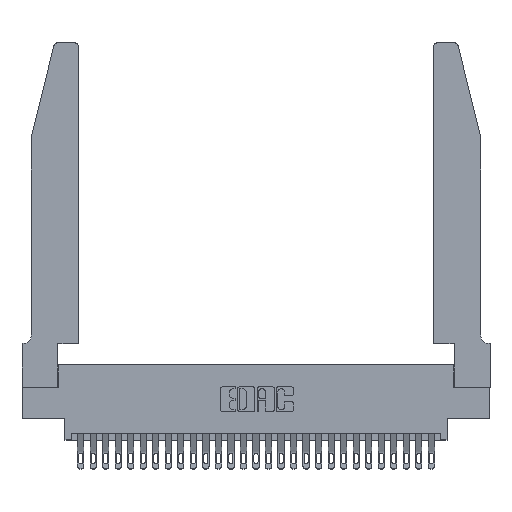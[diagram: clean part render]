
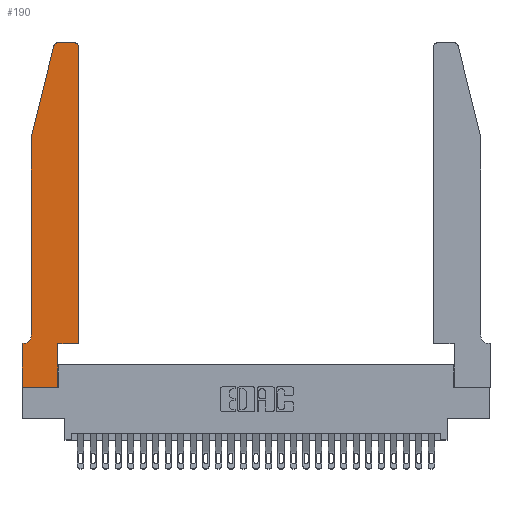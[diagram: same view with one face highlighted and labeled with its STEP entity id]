
A CAD part, top view. The second image highlights one B-rep face of the part: STEP entity #190.
In plain terms, the highlighted planar face has unit normal (0, 0, 1).
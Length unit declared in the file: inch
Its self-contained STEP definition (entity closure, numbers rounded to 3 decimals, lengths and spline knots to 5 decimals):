
#25 = ORIENTED_EDGE ( 'NONE', *, *, #14336, .T. ) ;
#148 = ORIENTED_EDGE ( 'NONE', *, *, #8840, .T. ) ;
#163 = EDGE_CURVE ( 'NONE', #23841, #16520, #17546, .T. ) ;
#190 = ADVANCED_FACE ( 'NONE', ( #3991 ), #472, .T. ) ;
#430 = VECTOR ( 'NONE', #6743, 39.37008 ) ;
#472 = PLANE ( 'NONE',  #8886 ) ;
#648 = CARTESIAN_POINT ( 'NONE',  ( 0.4505, 0.35, 0.37 ) ) ;
#1099 = EDGE_CURVE ( 'NONE', #1543, #5972, #5007, .T. ) ;
#1498 = LINE ( 'NONE', #7025, #430 ) ;
#1543 = VERTEX_POINT ( 'NONE', #26610 ) ;
#1707 = CARTESIAN_POINT ( 'NONE',  ( 0.2605, 2.75, 0.37 ) ) ;
#2311 = DIRECTION ( 'NONE',  ( 1., 0., 0. ) ) ;
#2401 = ORIENTED_EDGE ( 'NONE', *, *, #26664, .T. ) ;
#3390 = VECTOR ( 'NONE', #27976, 39.37008 ) ;
#3510 = DIRECTION ( 'NONE',  ( 0., 0., 1. ) ) ;
#3991 = FACE_OUTER_BOUND ( 'NONE', #22065, .T. ) ;
#4996 = EDGE_CURVE ( 'NONE', #13910, #7833, #11927, .T. ) ;
#5005 = CARTESIAN_POINT ( 'NONE',  ( 0.0755, 0.35, 0.37 ) ) ;
#5007 = CIRCLE ( 'NONE', #23324, 0.07 ) ;
#5354 = CIRCLE ( 'NONE', #14340, 0.03 ) ;
#5479 = VERTEX_POINT ( 'NONE', #13765 ) ;
#5972 = VERTEX_POINT ( 'NONE', #24914 ) ;
#6438 = DIRECTION ( 'NONE',  ( 0., -1., 0. ) ) ;
#6489 = VERTEX_POINT ( 'NONE', #14662 ) ;
#6595 = CARTESIAN_POINT ( 'NONE',  ( 0., 0.35, 0.37 ) ) ;
#6743 = DIRECTION ( 'NONE',  ( 0., -1., 0. ) ) ;
#6972 = EDGE_CURVE ( 'NONE', #5479, #14205, #20443, .T. ) ;
#7025 = CARTESIAN_POINT ( 'NONE',  ( 0., 0., 0.37 ) ) ;
#7113 = LINE ( 'NONE', #24559, #20734 ) ;
#7833 = VERTEX_POINT ( 'NONE', #26004 ) ;
#8429 = VECTOR ( 'NONE', #21575, 39.37008 ) ;
#8840 = EDGE_CURVE ( 'NONE', #16288, #6489, #14554, .T. ) ;
#8886 = AXIS2_PLACEMENT_3D ( 'NONE', #12289, #14259, #19126 ) ;
#8894 = EDGE_CURVE ( 'NONE', #14205, #1543, #14892, .T. ) ;
#8908 = CARTESIAN_POINT ( 'NONE',  ( 0.0055, 0.42, 0.37 ) ) ;
#9817 = EDGE_CURVE ( 'NONE', #5972, #24705, #28520, .T. ) ;
#9888 = CARTESIAN_POINT ( 'NONE',  ( 0., 0., 0.37 ) ) ;
#11049 = CARTESIAN_POINT ( 'NONE',  ( 0.0755, 2., 0.37 ) ) ;
#11228 = DIRECTION ( 'NONE',  ( 0., 0., -1. ) ) ;
#11453 = ORIENTED_EDGE ( 'NONE', *, *, #4996, .T. ) ;
#11559 = VECTOR ( 'NONE', #13982, 39.37008 ) ;
#11583 = DIRECTION ( 'NONE',  ( 0., 1., 0. ) ) ;
#11827 = DIRECTION ( 'NONE',  ( 1., 0., 0. ) ) ;
#11927 = LINE ( 'NONE', #13743, #27342 ) ;
#11958 = CARTESIAN_POINT ( 'NONE',  ( 0.2865, 0.35, 0.37 ) ) ;
#12289 = CARTESIAN_POINT ( 'NONE',  ( 0., 0.35, 0.37 ) ) ;
#12913 = CARTESIAN_POINT ( 'NONE',  ( 0.284, 2.72, 0.37 ) ) ;
#13577 = EDGE_CURVE ( 'NONE', #6489, #5479, #5354, .T. ) ;
#13691 = CARTESIAN_POINT ( 'NONE',  ( 0.4205, 2.75, 0.37 ) ) ;
#13743 = CARTESIAN_POINT ( 'NONE',  ( 0.4505, 0.35, 0.37 ) ) ;
#13765 = CARTESIAN_POINT ( 'NONE',  ( 0.25487, 2.72718, 0.37 ) ) ;
#13788 = DIRECTION ( 'NONE',  ( -1., 0., 0. ) ) ;
#13910 = VERTEX_POINT ( 'NONE', #648 ) ;
#13982 = DIRECTION ( 'NONE',  ( 0., 1., 0. ) ) ;
#14205 = VERTEX_POINT ( 'NONE', #28058 ) ;
#14259 = DIRECTION ( 'NONE',  ( 0., 0., 1. ) ) ;
#14336 = EDGE_CURVE ( 'NONE', #21540, #23841, #15957, .T. ) ;
#14340 = AXIS2_PLACEMENT_3D ( 'NONE', #12913, #3510, #23954 ) ;
#14554 = LINE ( 'NONE', #1707, #19160 ) ;
#14662 = CARTESIAN_POINT ( 'NONE',  ( 0.284, 2.75, 0.37 ) ) ;
#14892 = LINE ( 'NONE', #11049, #26388 ) ;
#15308 = CIRCLE ( 'NONE', #25494, 0.03 ) ;
#15957 = LINE ( 'NONE', #9888, #8429 ) ;
#16288 = VERTEX_POINT ( 'NONE', #13691 ) ;
#16520 = VERTEX_POINT ( 'NONE', #11958 ) ;
#16602 = ORIENTED_EDGE ( 'NONE', *, *, #1099, .T. ) ;
#17546 = LINE ( 'NONE', #20794, #11559 ) ;
#18133 = ORIENTED_EDGE ( 'NONE', *, *, #163, .T. ) ;
#18179 = ORIENTED_EDGE ( 'NONE', *, *, #6972, .T. ) ;
#18992 = CARTESIAN_POINT ( 'NONE',  ( 0.2865, 0., 0.37 ) ) ;
#19126 = DIRECTION ( 'NONE',  ( 1., 0., 0. ) ) ;
#19160 = VECTOR ( 'NONE', #20001, 39.37008 ) ;
#19374 = DIRECTION ( 'NONE',  ( -0.239, -0.971, 0. ) ) ;
#19574 = CARTESIAN_POINT ( 'NONE',  ( 0.0755, 2., 0.37 ) ) ;
#19671 = VECTOR ( 'NONE', #19374, 39.37008 ) ;
#20001 = DIRECTION ( 'NONE',  ( -1., 0., 0. ) ) ;
#20443 = LINE ( 'NONE', #19574, #19671 ) ;
#20734 = VECTOR ( 'NONE', #2311, 39.37008 ) ;
#20794 = CARTESIAN_POINT ( 'NONE',  ( 0.2865, 0.35, 0.37 ) ) ;
#21540 = VERTEX_POINT ( 'NONE', #22901 ) ;
#21575 = DIRECTION ( 'NONE',  ( 1., 0., 0. ) ) ;
#22065 = EDGE_LOOP ( 'NONE', ( #148, #28515, #18179, #25093, #16602, #25473, #2401, #25, #18133, #28893, #11453, #22717 ) ) ;
#22591 = EDGE_CURVE ( 'NONE', #16520, #13910, #7113, .T. ) ;
#22717 = ORIENTED_EDGE ( 'NONE', *, *, #22858, .T. ) ;
#22858 = EDGE_CURVE ( 'NONE', #7833, #16288, #15308, .T. ) ;
#22901 = CARTESIAN_POINT ( 'NONE',  ( 0., 0., 0.37 ) ) ;
#23324 = AXIS2_PLACEMENT_3D ( 'NONE', #8908, #11228, #13788 ) ;
#23841 = VERTEX_POINT ( 'NONE', #18992 ) ;
#23954 = DIRECTION ( 'NONE',  ( 1., 0., 0. ) ) ;
#24559 = CARTESIAN_POINT ( 'NONE',  ( 0.4505, 0.35, 0.37 ) ) ;
#24705 = VERTEX_POINT ( 'NONE', #6595 ) ;
#24914 = CARTESIAN_POINT ( 'NONE',  ( 0.0055, 0.35, 0.37 ) ) ;
#25093 = ORIENTED_EDGE ( 'NONE', *, *, #8894, .T. ) ;
#25473 = ORIENTED_EDGE ( 'NONE', *, *, #9817, .T. ) ;
#25494 = AXIS2_PLACEMENT_3D ( 'NONE', #25831, #25529, #11827 ) ;
#25529 = DIRECTION ( 'NONE',  ( 0., 0., 1. ) ) ;
#25831 = CARTESIAN_POINT ( 'NONE',  ( 0.4205, 2.72, 0.37 ) ) ;
#26004 = CARTESIAN_POINT ( 'NONE',  ( 0.4505, 2.72, 0.37 ) ) ;
#26388 = VECTOR ( 'NONE', #6438, 39.37008 ) ;
#26610 = CARTESIAN_POINT ( 'NONE',  ( 0.0755, 0.42, 0.37 ) ) ;
#26664 = EDGE_CURVE ( 'NONE', #24705, #21540, #1498, .T. ) ;
#27342 = VECTOR ( 'NONE', #11583, 39.37008 ) ;
#27976 = DIRECTION ( 'NONE',  ( -1., 0., 0. ) ) ;
#28058 = CARTESIAN_POINT ( 'NONE',  ( 0.0755, 2., 0.37 ) ) ;
#28515 = ORIENTED_EDGE ( 'NONE', *, *, #13577, .T. ) ;
#28520 = LINE ( 'NONE', #5005, #3390 ) ;
#28893 = ORIENTED_EDGE ( 'NONE', *, *, #22591, .T. ) ;
